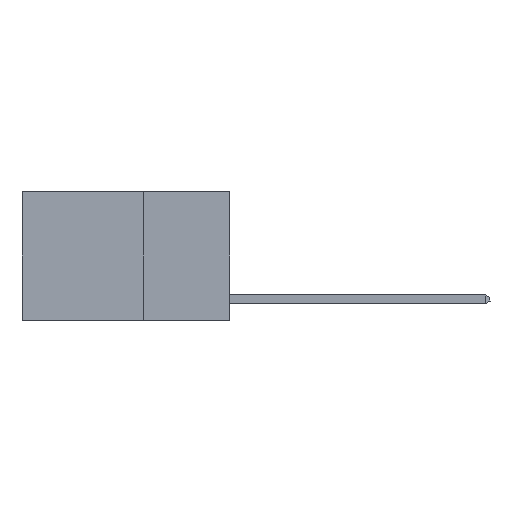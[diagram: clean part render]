
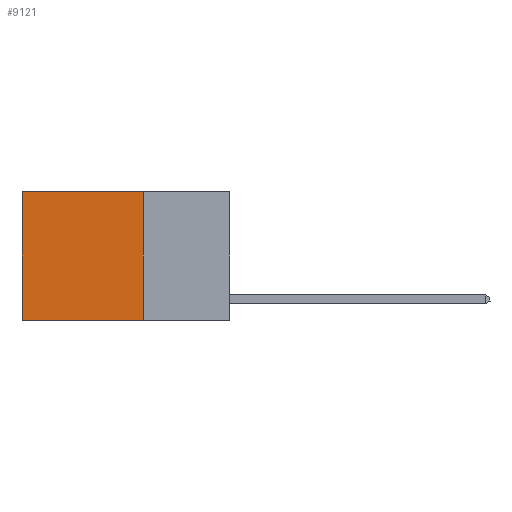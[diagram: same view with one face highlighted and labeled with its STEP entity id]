
A CAD part, left-side view. The second image highlights one B-rep face of the part: STEP entity #9121.
In plain terms, the highlighted planar face has unit normal (-1, 0, 0).
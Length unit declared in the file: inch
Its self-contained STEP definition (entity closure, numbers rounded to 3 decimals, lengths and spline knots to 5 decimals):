
#254 = AXIS2_PLACEMENT_3D ( 'NONE', #12334, #19504, #660 ) ;
#574 = ORIENTED_EDGE ( 'NONE', *, *, #13846, .T. ) ;
#660 = DIRECTION ( 'NONE',  ( 0., 0., -1. ) ) ;
#1123 = LINE ( 'NONE', #21660, #20981 ) ;
#2876 = VERTEX_POINT ( 'NONE', #19402 ) ;
#4195 = CARTESIAN_POINT ( 'NONE',  ( 0.2625, 0.6, -0.37 ) ) ;
#5541 = PLANE ( 'NONE',  #254 ) ;
#7073 = EDGE_CURVE ( 'NONE', #2876, #17709, #7967, .T. ) ;
#7466 = ORIENTED_EDGE ( 'NONE', *, *, #7073, .F. ) ;
#7967 = LINE ( 'NONE', #20112, #15557 ) ;
#9015 = DIRECTION ( 'NONE',  ( 0., 0., -1. ) ) ;
#9121 = ADVANCED_FACE ( 'NONE', ( #21416 ), #5541, .F. ) ;
#10135 = VECTOR ( 'NONE', #9015, 39.37008 ) ;
#10618 = CARTESIAN_POINT ( 'NONE',  ( 0.2625, 0.6, 0. ) ) ;
#10975 = ORIENTED_EDGE ( 'NONE', *, *, #20095, .T. ) ;
#11436 = DIRECTION ( 'NONE',  ( 0., 0., -1. ) ) ;
#12334 = CARTESIAN_POINT ( 'NONE',  ( 0.2625, 0.25, 0. ) ) ;
#12676 = LINE ( 'NONE', #21212, #15725 ) ;
#13180 = EDGE_CURVE ( 'NONE', #15281, #2876, #1123, .T. ) ;
#13846 = EDGE_CURVE ( 'NONE', #18505, #17709, #15920, .T. ) ;
#13988 = CARTESIAN_POINT ( 'NONE',  ( 0.2625, 0.6, 0. ) ) ;
#14628 = DIRECTION ( 'NONE',  ( 0., 1., 0. ) ) ;
#15281 = VERTEX_POINT ( 'NONE', #17221 ) ;
#15557 = VECTOR ( 'NONE', #14628, 39.37008 ) ;
#15725 = VECTOR ( 'NONE', #19312, 39.37008 ) ;
#15879 = ORIENTED_EDGE ( 'NONE', *, *, #13180, .F. ) ;
#15920 = LINE ( 'NONE', #10618, #10135 ) ;
#17221 = CARTESIAN_POINT ( 'NONE',  ( 0.2625, 0.25, 0. ) ) ;
#17709 = VERTEX_POINT ( 'NONE', #4195 ) ;
#18505 = VERTEX_POINT ( 'NONE', #13988 ) ;
#19312 = DIRECTION ( 'NONE',  ( 0., 1., 0. ) ) ;
#19402 = CARTESIAN_POINT ( 'NONE',  ( 0.2625, 0.25, -0.37 ) ) ;
#19504 = DIRECTION ( 'NONE',  ( 1., 0., 0. ) ) ;
#20095 = EDGE_CURVE ( 'NONE', #15281, #18505, #12676, .T. ) ;
#20112 = CARTESIAN_POINT ( 'NONE',  ( 0.2625, 0.25, -0.37 ) ) ;
#20837 = EDGE_LOOP ( 'NONE', ( #574, #7466, #15879, #10975 ) ) ;
#20981 = VECTOR ( 'NONE', #11436, 39.37008 ) ;
#21212 = CARTESIAN_POINT ( 'NONE',  ( 0.2625, 0.25, 0. ) ) ;
#21416 = FACE_OUTER_BOUND ( 'NONE', #20837, .T. ) ;
#21660 = CARTESIAN_POINT ( 'NONE',  ( 0.2625, 0.25, 0. ) ) ;
